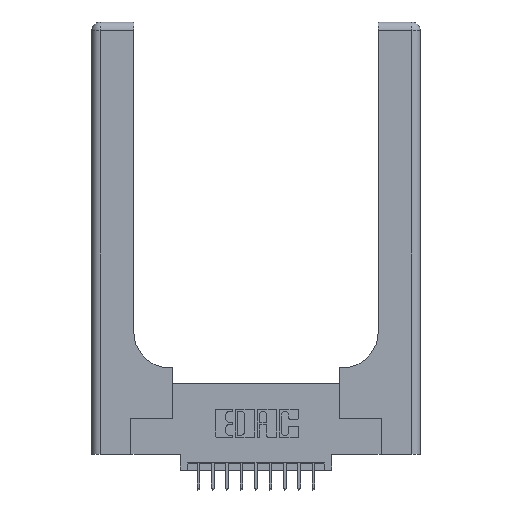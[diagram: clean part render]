
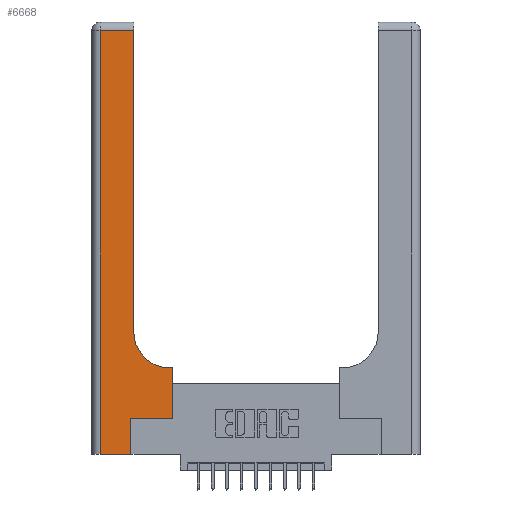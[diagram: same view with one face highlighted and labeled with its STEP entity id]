
A CAD part, top view. The second image highlights one B-rep face of the part: STEP entity #6668.
In plain terms, the highlighted planar face has unit normal (0, 0, 1).
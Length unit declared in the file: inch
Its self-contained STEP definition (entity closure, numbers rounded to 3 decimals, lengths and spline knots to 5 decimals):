
#130 = VERTEX_POINT ( 'NONE', #16293 ) ;
#145 = VECTOR ( 'NONE', #15625, 39.37008 ) ;
#163 = EDGE_CURVE ( 'NONE', #12181, #1574, #13259, .T. ) ;
#548 = DIRECTION ( 'NONE',  ( 1., 0., 0. ) ) ;
#583 = CARTESIAN_POINT ( 'NONE',  ( 0.5585, 0.25, 0.37 ) ) ;
#589 = CARTESIAN_POINT ( 'NONE',  ( 0.5585, 0.25, 0.37 ) ) ;
#1574 = VERTEX_POINT ( 'NONE', #9326 ) ;
#1752 = EDGE_CURVE ( 'NONE', #1574, #5817, #3975, .T. ) ;
#2142 = CARTESIAN_POINT ( 'NONE',  ( 0.2915, 0.6, 0.37 ) ) ;
#2152 = VECTOR ( 'NONE', #548, 39.37008 ) ;
#2523 = CARTESIAN_POINT ( 'NONE',  ( 0.2915, 3., 0.37 ) ) ;
#2900 = VERTEX_POINT ( 'NONE', #13667 ) ;
#2908 = DIRECTION ( 'NONE',  ( -1., 0., 0. ) ) ;
#3495 = EDGE_LOOP ( 'NONE', ( #6103, #14162, #6629, #7149, #15859, #15181, #11824, #16031, #16501 ) ) ;
#3756 = VECTOR ( 'NONE', #10345, 39.37008 ) ;
#3939 = CARTESIAN_POINT ( 'NONE',  ( 0.269, 0.25, 0.37 ) ) ;
#3975 = LINE ( 'NONE', #7998, #3756 ) ;
#4046 = VECTOR ( 'NONE', #6167, 39.37008 ) ;
#4054 = CARTESIAN_POINT ( 'NONE',  ( 0.06, 0., 0.37 ) ) ;
#4273 = EDGE_CURVE ( 'NONE', #11154, #130, #10218, .T. ) ;
#4382 = CARTESIAN_POINT ( 'NONE',  ( 0., 0., 0.37 ) ) ;
#4477 = DIRECTION ( 'NONE',  ( 0., -1., 0. ) ) ;
#4569 = EDGE_CURVE ( 'NONE', #5817, #10462, #14929, .T. ) ;
#4756 = VECTOR ( 'NONE', #16265, 39.37008 ) ;
#4959 = CARTESIAN_POINT ( 'NONE',  ( 0.269, 0.25, 0.37 ) ) ;
#5067 = EDGE_CURVE ( 'NONE', #130, #8993, #5987, .T. ) ;
#5311 = CARTESIAN_POINT ( 'NONE',  ( 0.5415, 0.85, 0.37 ) ) ;
#5737 = EDGE_CURVE ( 'NONE', #12633, #2900, #9212, .T. ) ;
#5817 = VERTEX_POINT ( 'NONE', #3939 ) ;
#5893 = PLANE ( 'NONE',  #9053 ) ;
#5987 = CIRCLE ( 'NONE', #15556, 0.25 ) ;
#6098 = VECTOR ( 'NONE', #8506, 39.37008 ) ;
#6103 = ORIENTED_EDGE ( 'NONE', *, *, #13173, .T. ) ;
#6167 = DIRECTION ( 'NONE',  ( -1., 0., 0. ) ) ;
#6528 = VECTOR ( 'NONE', #2908, 39.37008 ) ;
#6629 = ORIENTED_EDGE ( 'NONE', *, *, #16477, .T. ) ;
#6668 = ADVANCED_FACE ( 'NONE', ( #8722 ), #5893, .F. ) ;
#6675 = DIRECTION ( 'NONE',  ( 1., 0., 0. ) ) ;
#6944 = LINE ( 'NONE', #14763, #15090 ) ;
#7149 = ORIENTED_EDGE ( 'NONE', *, *, #163, .T. ) ;
#7998 = CARTESIAN_POINT ( 'NONE',  ( 0.269, 0., 0.37 ) ) ;
#8063 = DIRECTION ( 'NONE',  ( 0., 0., -1. ) ) ;
#8506 = DIRECTION ( 'NONE',  ( 1., 0., 0. ) ) ;
#8722 = FACE_OUTER_BOUND ( 'NONE', #3495, .T. ) ;
#8993 = VERTEX_POINT ( 'NONE', #15259 ) ;
#9053 = AXIS2_PLACEMENT_3D ( 'NONE', #11150, #13951, #16339 ) ;
#9212 = LINE ( 'NONE', #14515, #6528 ) ;
#9326 = CARTESIAN_POINT ( 'NONE',  ( 0.269, 0., 0.37 ) ) ;
#10218 = LINE ( 'NONE', #2142, #4046 ) ;
#10345 = DIRECTION ( 'NONE',  ( 0., 1., 0. ) ) ;
#10462 = VERTEX_POINT ( 'NONE', #583 ) ;
#11150 = CARTESIAN_POINT ( 'NONE',  ( 0., 3., 0.37 ) ) ;
#11154 = VERTEX_POINT ( 'NONE', #13480 ) ;
#11824 = ORIENTED_EDGE ( 'NONE', *, *, #12567, .T. ) ;
#12181 = VERTEX_POINT ( 'NONE', #4054 ) ;
#12257 = CARTESIAN_POINT ( 'NONE',  ( 0.2915, 2.94, 0.37 ) ) ;
#12567 = EDGE_CURVE ( 'NONE', #10462, #11154, #14814, .T. ) ;
#12633 = VERTEX_POINT ( 'NONE', #12257 ) ;
#13173 = EDGE_CURVE ( 'NONE', #8993, #12633, #14277, .T. ) ;
#13259 = LINE ( 'NONE', #4382, #6098 ) ;
#13480 = CARTESIAN_POINT ( 'NONE',  ( 0.5585, 0.6, 0.37 ) ) ;
#13667 = CARTESIAN_POINT ( 'NONE',  ( 0.06, 2.94, 0.37 ) ) ;
#13951 = DIRECTION ( 'NONE',  ( 0., 0., -1. ) ) ;
#14162 = ORIENTED_EDGE ( 'NONE', *, *, #5737, .T. ) ;
#14277 = LINE ( 'NONE', #2523, #145 ) ;
#14515 = CARTESIAN_POINT ( 'NONE',  ( 0., 2.94, 0.37 ) ) ;
#14763 = CARTESIAN_POINT ( 'NONE',  ( 0.06, 3., 0.37 ) ) ;
#14814 = LINE ( 'NONE', #589, #4756 ) ;
#14929 = LINE ( 'NONE', #4959, #2152 ) ;
#15090 = VECTOR ( 'NONE', #4477, 39.37008 ) ;
#15181 = ORIENTED_EDGE ( 'NONE', *, *, #4569, .T. ) ;
#15259 = CARTESIAN_POINT ( 'NONE',  ( 0.2915, 0.85, 0.37 ) ) ;
#15556 = AXIS2_PLACEMENT_3D ( 'NONE', #5311, #8063, #6675 ) ;
#15625 = DIRECTION ( 'NONE',  ( 0., 1., 0. ) ) ;
#15859 = ORIENTED_EDGE ( 'NONE', *, *, #1752, .T. ) ;
#16031 = ORIENTED_EDGE ( 'NONE', *, *, #4273, .T. ) ;
#16265 = DIRECTION ( 'NONE',  ( 0., 1., 0. ) ) ;
#16293 = CARTESIAN_POINT ( 'NONE',  ( 0.5415, 0.6, 0.37 ) ) ;
#16339 = DIRECTION ( 'NONE',  ( -1., 0., 0. ) ) ;
#16477 = EDGE_CURVE ( 'NONE', #2900, #12181, #6944, .T. ) ;
#16501 = ORIENTED_EDGE ( 'NONE', *, *, #5067, .T. ) ;
